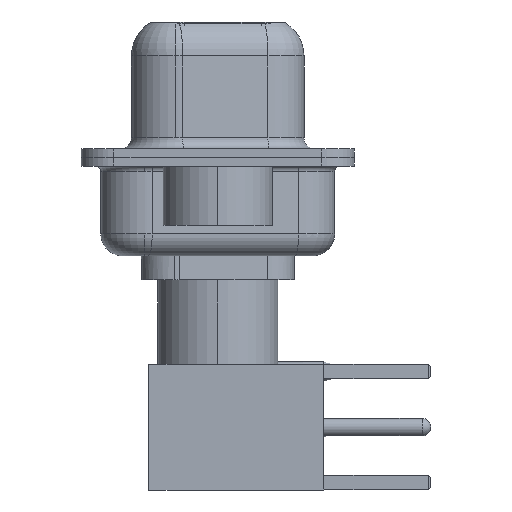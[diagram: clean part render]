
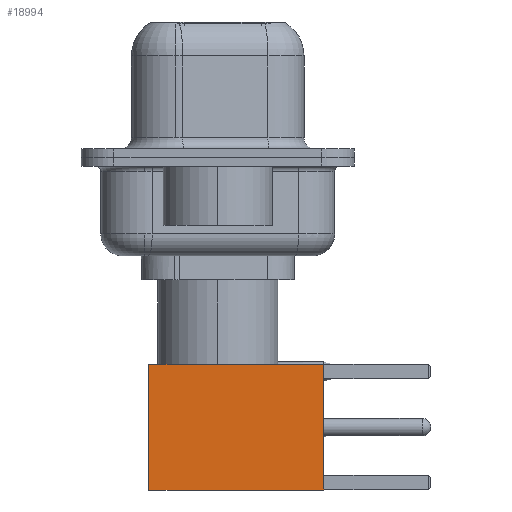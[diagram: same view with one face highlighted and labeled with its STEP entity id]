
A CAD part, left-side view. The second image highlights one B-rep face of the part: STEP entity #18994.
In plain terms, the highlighted face is planar.
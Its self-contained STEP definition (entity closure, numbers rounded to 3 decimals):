
#38 = CARTESIAN_POINT ( 'NONE',  ( -2.875, 2.875, 0. ) ) ;
#405 = VECTOR ( 'NONE', #17301, 1000. ) ;
#1028 = VERTEX_POINT ( 'NONE', #17319 ) ;
#1060 = DIRECTION ( 'NONE',  ( 0., 0., 1. ) ) ;
#1161 = DIRECTION ( 'NONE',  ( 0., 1., 0. ) ) ;
#1740 = CARTESIAN_POINT ( 'NONE',  ( 0., 2.875, 8. ) ) ;
#1874 = DIRECTION ( 'NONE',  ( 0., 0., -1. ) ) ;
#3176 = LINE ( 'NONE', #1740, #12876 ) ;
#3645 = EDGE_CURVE ( 'NONE', #11580, #12482, #4795, .T. ) ;
#3783 = CARTESIAN_POINT ( 'NONE',  ( 2.875, 2.875, 0. ) ) ;
#4795 = LINE ( 'NONE', #19240, #405 ) ;
#5454 = CARTESIAN_POINT ( 'NONE',  ( -2.875, 2.875, 8. ) ) ;
#5497 = EDGE_CURVE ( 'NONE', #1028, #6092, #3176, .T. ) ;
#5660 = ORIENTED_EDGE ( 'NONE', *, *, #17757, .F. ) ;
#6092 = VERTEX_POINT ( 'NONE', #5454 ) ;
#6258 = VECTOR ( 'NONE', #19159, 1000. ) ;
#6647 = LINE ( 'NONE', #16077, #6258 ) ;
#8251 = ORIENTED_EDGE ( 'NONE', *, *, #5497, .F. ) ;
#10043 = CARTESIAN_POINT ( 'NONE',  ( 2.875, 2.875, 0. ) ) ;
#10909 = EDGE_CURVE ( 'NONE', #1028, #11580, #15897, .T. ) ;
#11033 = VECTOR ( 'NONE', #1874, 1000. ) ;
#11580 = VERTEX_POINT ( 'NONE', #3783 ) ;
#12160 = ORIENTED_EDGE ( 'NONE', *, *, #10909, .T. ) ;
#12482 = VERTEX_POINT ( 'NONE', #38 ) ;
#12876 = VECTOR ( 'NONE', #15462, 1000. ) ;
#14093 = ORIENTED_EDGE ( 'NONE', *, *, #3645, .T. ) ;
#15073 = CARTESIAN_POINT ( 'NONE',  ( 2.875, 2.875, 0. ) ) ;
#15462 = DIRECTION ( 'NONE',  ( -1., 0., 0. ) ) ;
#15897 = LINE ( 'NONE', #10043, #11033 ) ;
#16051 = AXIS2_PLACEMENT_3D ( 'NONE', #15073, #1161, #1060 ) ;
#16077 = CARTESIAN_POINT ( 'NONE',  ( -2.875, 2.875, 0. ) ) ;
#16721 = PLANE ( 'NONE',  #16051 ) ;
#17301 = DIRECTION ( 'NONE',  ( -1., 0., 0. ) ) ;
#17319 = CARTESIAN_POINT ( 'NONE',  ( 2.875, 2.875, 8. ) ) ;
#17757 = EDGE_CURVE ( 'NONE', #6092, #12482, #6647, .T. ) ;
#18994 = ADVANCED_FACE ( 'NONE', ( #19997 ), #16721, .T. ) ;
#19159 = DIRECTION ( 'NONE',  ( 0., 0., -1. ) ) ;
#19240 = CARTESIAN_POINT ( 'NONE',  ( 0., 2.875, 0. ) ) ;
#19892 = EDGE_LOOP ( 'NONE', ( #12160, #14093, #5660, #8251 ) ) ;
#19997 = FACE_OUTER_BOUND ( 'NONE', #19892, .T. ) ;
